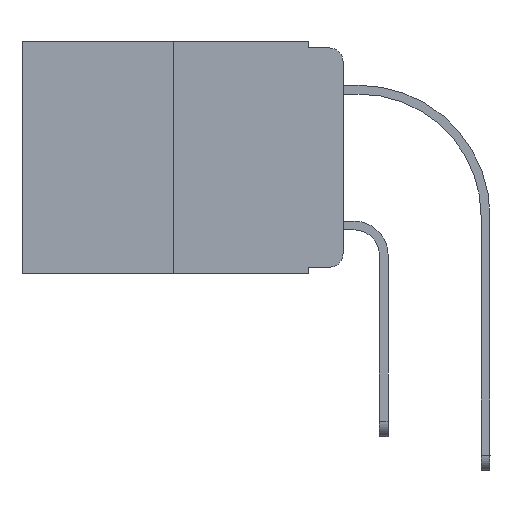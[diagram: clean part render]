
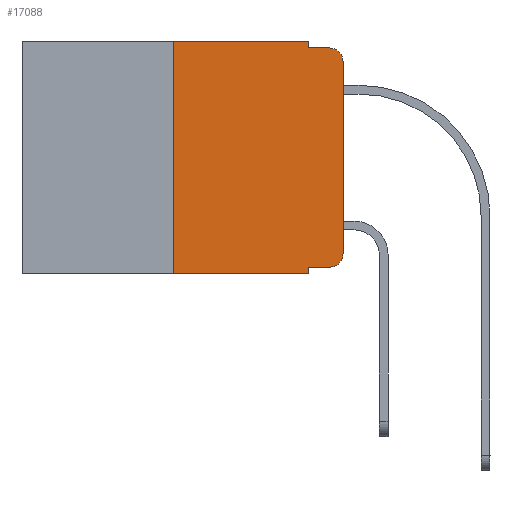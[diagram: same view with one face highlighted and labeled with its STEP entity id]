
A CAD part, left-side view. The second image highlights one B-rep face of the part: STEP entity #17088.
In plain terms, the highlighted planar face has unit normal (-1, 0, 0).
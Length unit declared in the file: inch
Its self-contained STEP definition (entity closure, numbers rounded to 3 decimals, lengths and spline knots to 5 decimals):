
#386 = EDGE_CURVE ( 'NONE', #545, #9569, #22283, .T. ) ;
#545 = VERTEX_POINT ( 'NONE', #13665 ) ;
#887 = LINE ( 'NONE', #17450, #22858 ) ;
#1009 = VERTEX_POINT ( 'NONE', #13994 ) ;
#1493 = EDGE_CURVE ( 'NONE', #1009, #3759, #2234, .T. ) ;
#1897 = CARTESIAN_POINT ( 'NONE',  ( 0., 0.051, -0.343 ) ) ;
#1979 = DIRECTION ( 'NONE',  ( 0., -1., 0. ) ) ;
#2234 = CIRCLE ( 'NONE', #9283, 0.02 ) ;
#2355 = DIRECTION ( 'NONE',  ( 0., -1., 0. ) ) ;
#2598 = ORIENTED_EDGE ( 'NONE', *, *, #14056, .F. ) ;
#2736 = EDGE_LOOP ( 'NONE', ( #7189, #18812, #6353, #18369, #6982, #2598, #6340, #17020, #17421, #13588 ) ) ;
#3086 = VECTOR ( 'NONE', #16482, 39.37008 ) ;
#3369 = CARTESIAN_POINT ( 'NONE',  ( 0., 0., 0. ) ) ;
#3759 = VERTEX_POINT ( 'NONE', #23251 ) ;
#3823 = LINE ( 'NONE', #18799, #21456 ) ;
#4041 = CARTESIAN_POINT ( 'NONE',  ( 0., 0.473, 0. ) ) ;
#4207 = EDGE_CURVE ( 'NONE', #11883, #1009, #4557, .T. ) ;
#4506 = DIRECTION ( 'NONE',  ( -1., 0., 0. ) ) ;
#4557 = LINE ( 'NONE', #19172, #18310 ) ;
#4879 = CARTESIAN_POINT ( 'NONE',  ( 0., 0.02, -0.313 ) ) ;
#4934 = EDGE_CURVE ( 'NONE', #20720, #19531, #21242, .T. ) ;
#5330 = DIRECTION ( 'NONE',  ( 1., 0., 0. ) ) ;
#6056 = AXIS2_PLACEMENT_3D ( 'NONE', #24251, #5330, #7293 ) ;
#6340 = ORIENTED_EDGE ( 'NONE', *, *, #386, .T. ) ;
#6353 = ORIENTED_EDGE ( 'NONE', *, *, #7461, .F. ) ;
#6502 = CARTESIAN_POINT ( 'NONE',  ( 0., 0.25, 0. ) ) ;
#6982 = ORIENTED_EDGE ( 'NONE', *, *, #4934, .F. ) ;
#7189 = ORIENTED_EDGE ( 'NONE', *, *, #18450, .T. ) ;
#7293 = DIRECTION ( 'NONE',  ( 0., 0., -1. ) ) ;
#7461 = EDGE_CURVE ( 'NONE', #20509, #10045, #3823, .T. ) ;
#8329 = VECTOR ( 'NONE', #11381, 39.37008 ) ;
#8362 = CARTESIAN_POINT ( 'NONE',  ( 0., 0.02, -0.01 ) ) ;
#8620 = VECTOR ( 'NONE', #9564, 39.37008 ) ;
#9245 = VECTOR ( 'NONE', #10866, 39.37008 ) ;
#9283 = AXIS2_PLACEMENT_3D ( 'NONE', #4879, #4506, #12003 ) ;
#9336 = LINE ( 'NONE', #16806, #8620 ) ;
#9564 = DIRECTION ( 'NONE',  ( 0., 0., -1. ) ) ;
#9569 = VERTEX_POINT ( 'NONE', #1897 ) ;
#9700 = DIRECTION ( 'NONE',  ( -1., 0., 0. ) ) ;
#9740 = VECTOR ( 'NONE', #19159, 39.37008 ) ;
#10045 = VERTEX_POINT ( 'NONE', #8362 ) ;
#10866 = DIRECTION ( 'NONE',  ( 0., 0., 1. ) ) ;
#11381 = DIRECTION ( 'NONE',  ( 0., 0., 1. ) ) ;
#11520 = DIRECTION ( 'NONE',  ( 0., 0., -1. ) ) ;
#11664 = EDGE_CURVE ( 'NONE', #11883, #9569, #9336, .T. ) ;
#11883 = VERTEX_POINT ( 'NONE', #16277 ) ;
#12003 = DIRECTION ( 'NONE',  ( 0., 0., -1. ) ) ;
#12688 = FACE_OUTER_BOUND ( 'NONE', #2736, .T. ) ;
#12694 = LINE ( 'NONE', #3369, #9245 ) ;
#13054 = PLANE ( 'NONE',  #6056 ) ;
#13396 = AXIS2_PLACEMENT_3D ( 'NONE', #17406, #9700, #11520 ) ;
#13572 = EDGE_CURVE ( 'NONE', #21491, #10045, #20849, .T. ) ;
#13588 = ORIENTED_EDGE ( 'NONE', *, *, #1493, .T. ) ;
#13665 = CARTESIAN_POINT ( 'NONE',  ( 0., 0.25, -0.343 ) ) ;
#13994 = CARTESIAN_POINT ( 'NONE',  ( 0., 0.02, -0.333 ) ) ;
#14056 = EDGE_CURVE ( 'NONE', #545, #20720, #15180, .T. ) ;
#14594 = CARTESIAN_POINT ( 'NONE',  ( 0., 0.051, -0.01 ) ) ;
#15180 = LINE ( 'NONE', #20719, #8329 ) ;
#15619 = DIRECTION ( 'NONE',  ( 0., 0., -1. ) ) ;
#16277 = CARTESIAN_POINT ( 'NONE',  ( 0., 0.051, -0.333 ) ) ;
#16424 = EDGE_CURVE ( 'NONE', #19531, #20509, #887, .T. ) ;
#16482 = DIRECTION ( 'NONE',  ( 0., -1., 0. ) ) ;
#16806 = CARTESIAN_POINT ( 'NONE',  ( 0., 0.051, 0. ) ) ;
#17020 = ORIENTED_EDGE ( 'NONE', *, *, #11664, .F. ) ;
#17088 = ADVANCED_FACE ( 'NONE', ( #12688 ), #13054, .F. ) ;
#17406 = CARTESIAN_POINT ( 'NONE',  ( 0., 0.02, -0.03 ) ) ;
#17421 = ORIENTED_EDGE ( 'NONE', *, *, #4207, .T. ) ;
#17450 = CARTESIAN_POINT ( 'NONE',  ( 0., 0.051, 0. ) ) ;
#17772 = CARTESIAN_POINT ( 'NONE',  ( 0., 0.051, 0. ) ) ;
#18310 = VECTOR ( 'NONE', #2355, 39.37008 ) ;
#18369 = ORIENTED_EDGE ( 'NONE', *, *, #16424, .F. ) ;
#18450 = EDGE_CURVE ( 'NONE', #3759, #21491, #12694, .T. ) ;
#18631 = CARTESIAN_POINT ( 'NONE',  ( 0., 0., -0.03 ) ) ;
#18799 = CARTESIAN_POINT ( 'NONE',  ( 0., 0.051, -0.01 ) ) ;
#18812 = ORIENTED_EDGE ( 'NONE', *, *, #13572, .T. ) ;
#19159 = DIRECTION ( 'NONE',  ( 0., -1., 0. ) ) ;
#19172 = CARTESIAN_POINT ( 'NONE',  ( 0., 0.051, -0.333 ) ) ;
#19531 = VERTEX_POINT ( 'NONE', #17772 ) ;
#20509 = VERTEX_POINT ( 'NONE', #14594 ) ;
#20719 = CARTESIAN_POINT ( 'NONE',  ( 0., 0.25, 0. ) ) ;
#20720 = VERTEX_POINT ( 'NONE', #6502 ) ;
#20849 = CIRCLE ( 'NONE', #13396, 0.02 ) ;
#21242 = LINE ( 'NONE', #4041, #9740 ) ;
#21456 = VECTOR ( 'NONE', #1979, 39.37008 ) ;
#21491 = VERTEX_POINT ( 'NONE', #18631 ) ;
#22143 = CARTESIAN_POINT ( 'NONE',  ( 0., 0.473, -0.343 ) ) ;
#22283 = LINE ( 'NONE', #22143, #3086 ) ;
#22858 = VECTOR ( 'NONE', #15619, 39.37008 ) ;
#23251 = CARTESIAN_POINT ( 'NONE',  ( 0., 0., -0.313 ) ) ;
#24251 = CARTESIAN_POINT ( 'NONE',  ( 0., 0.473, 0. ) ) ;
